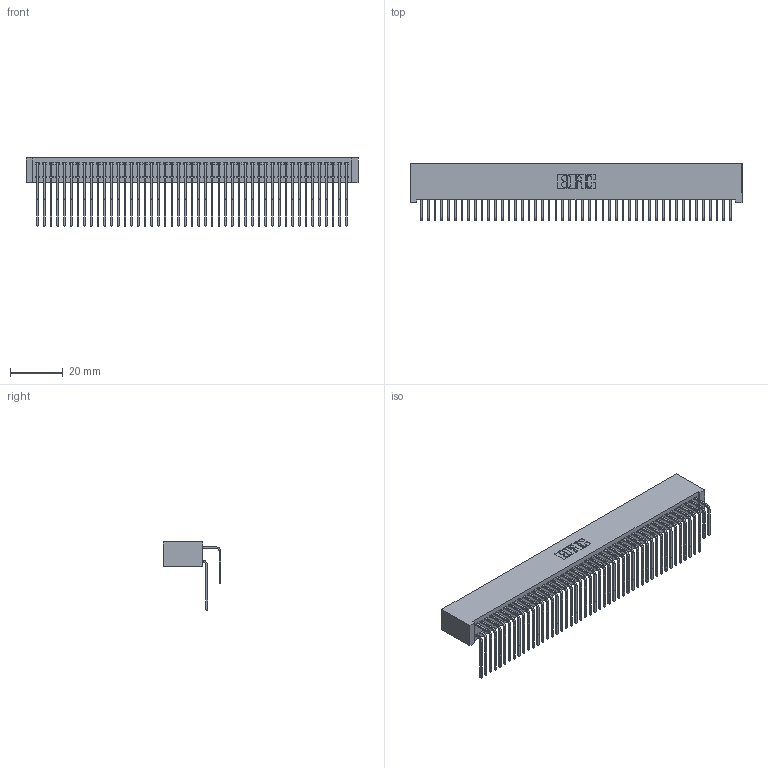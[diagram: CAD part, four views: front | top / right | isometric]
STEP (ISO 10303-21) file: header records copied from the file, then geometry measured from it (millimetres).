
FILE_DESCRIPTION (( 'STEP AP203' ), '1' );
FILE_NAME ('392-094-558-201.STEP', '2018-08-18T09:16:32', ( '' ), ( '' ), 'SwSTEP 2.0', 'SolidWorks 2016', '' );
FILE_SCHEMA (( 'CONFIG_CONTROL_DESIGN' ));
Length unit declared in the file: inch
Products named in the file (4): 342 Part_Lugless; 345-292-001_558 559 Tail - 1; 345-292-001_558 Tail - 2; 392-094-558-201
Assembly tree (95 placements, depth 2):
  392-094-558-201
    342 Part_Lugless
    345-292-001_558 559 Tail - 1  x47
    345-292-001_558 Tail - 2  x47
Bounding box: 125.63 x 21.91 x 25.78 mm (x, y, z)
Volume: 12293.1 mm3; surface area: 23032.6 mm2
Topology: 95 solids, 95 shells, 5178 faces, 15409 edges, 10146 vertices
Faces by surface type: plane 3634, cylinder 1544
Entity records: 30965 total; most frequent: CARTESIAN_POINT 5173, ORIENTED_EDGE 5058, DIRECTION 4385, EDGE_CURVE 2529, VECTOR 2369, LINE 2369, VERTEX_POINT 1682, AXIS2_PLACEMENT_3D 1008
